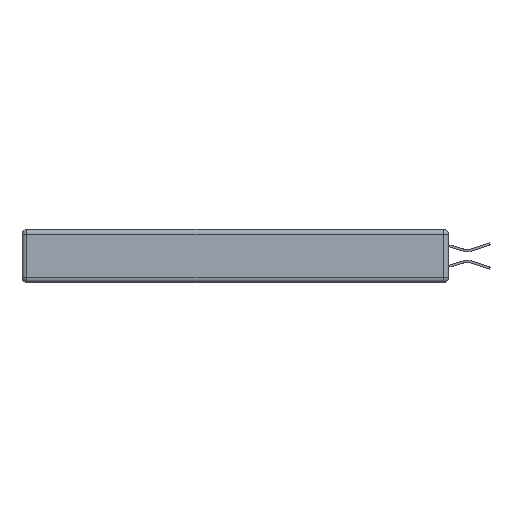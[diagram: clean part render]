
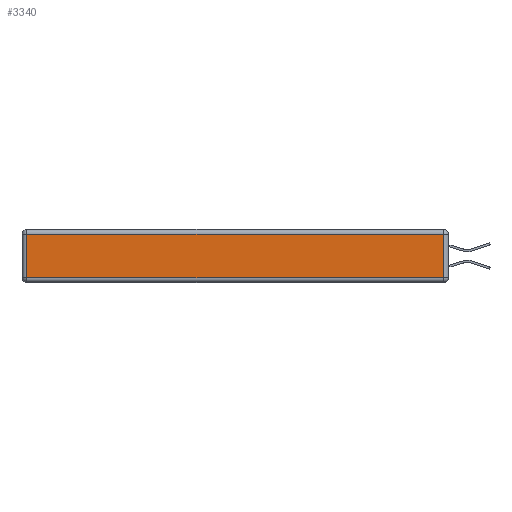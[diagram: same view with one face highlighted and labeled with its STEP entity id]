
A CAD part, left-side view. The second image highlights one B-rep face of the part: STEP entity #3340.
In plain terms, the highlighted planar face has unit normal (-1, 0, 0).
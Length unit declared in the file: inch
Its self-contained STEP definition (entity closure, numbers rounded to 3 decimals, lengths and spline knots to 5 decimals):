
#160 = FACE_OUTER_BOUND ( 'NONE', #12454, .T. ) ;
#816 = EDGE_CURVE ( 'NONE', #9520, #9912, #14192, .T. ) ;
#1894 = VECTOR ( 'NONE', #7709, 39.37008 ) ;
#2369 = EDGE_CURVE ( 'NONE', #10265, #9520, #4053, .T. ) ;
#2679 = CARTESIAN_POINT ( 'NONE',  ( 0., 0.03, -0.313 ) ) ;
#3340 = ADVANCED_FACE ( 'NONE', ( #160 ), #10654, .T. ) ;
#3723 = LINE ( 'NONE', #14735, #1894 ) ;
#3736 = DIRECTION ( 'NONE',  ( -1., 0., 0. ) ) ;
#3776 = ORIENTED_EDGE ( 'NONE', *, *, #7229, .T. ) ;
#4053 = LINE ( 'NONE', #13322, #5335 ) ;
#4878 = CARTESIAN_POINT ( 'NONE',  ( 0., 0., -0.343 ) ) ;
#5335 = VECTOR ( 'NONE', #8555, 39.37008 ) ;
#6012 = VERTEX_POINT ( 'NONE', #2679 ) ;
#6116 = CARTESIAN_POINT ( 'NONE',  ( 0., 2.72, -0.03 ) ) ;
#6120 = VECTOR ( 'NONE', #7232, 39.37008 ) ;
#6681 = LINE ( 'NONE', #7833, #11110 ) ;
#6700 = AXIS2_PLACEMENT_3D ( 'NONE', #4878, #3736, #7152 ) ;
#7152 = DIRECTION ( 'NONE',  ( 0., 0., 1. ) ) ;
#7221 = CARTESIAN_POINT ( 'NONE',  ( 0., 2.72, -0.313 ) ) ;
#7229 = EDGE_CURVE ( 'NONE', #6012, #10265, #3723, .T. ) ;
#7232 = DIRECTION ( 'NONE',  ( 0., 0., -1. ) ) ;
#7233 = ORIENTED_EDGE ( 'NONE', *, *, #8303, .T. ) ;
#7329 = ORIENTED_EDGE ( 'NONE', *, *, #816, .T. ) ;
#7709 = DIRECTION ( 'NONE',  ( 0., 0., 1. ) ) ;
#7833 = CARTESIAN_POINT ( 'NONE',  ( 0., 0., -0.313 ) ) ;
#8303 = EDGE_CURVE ( 'NONE', #9912, #6012, #6681, .T. ) ;
#8555 = DIRECTION ( 'NONE',  ( 0., 1., 0. ) ) ;
#9520 = VERTEX_POINT ( 'NONE', #6116 ) ;
#9912 = VERTEX_POINT ( 'NONE', #7221 ) ;
#10265 = VERTEX_POINT ( 'NONE', #13598 ) ;
#10654 = PLANE ( 'NONE',  #6700 ) ;
#11110 = VECTOR ( 'NONE', #14336, 39.37008 ) ;
#12454 = EDGE_LOOP ( 'NONE', ( #7233, #3776, #12458, #7329 ) ) ;
#12458 = ORIENTED_EDGE ( 'NONE', *, *, #2369, .T. ) ;
#13322 = CARTESIAN_POINT ( 'NONE',  ( 0., 2.75, -0.03 ) ) ;
#13598 = CARTESIAN_POINT ( 'NONE',  ( 0., 0.03, -0.03 ) ) ;
#14192 = LINE ( 'NONE', #15136, #6120 ) ;
#14336 = DIRECTION ( 'NONE',  ( 0., -1., 0. ) ) ;
#14735 = CARTESIAN_POINT ( 'NONE',  ( 0., 0.03, -0.343 ) ) ;
#15136 = CARTESIAN_POINT ( 'NONE',  ( 0., 2.72, -0.343 ) ) ;
